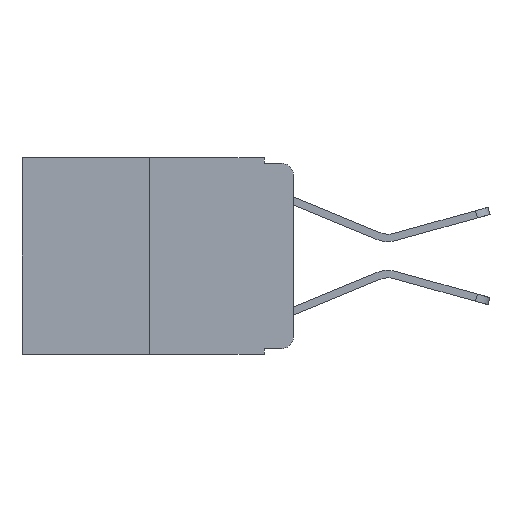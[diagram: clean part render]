
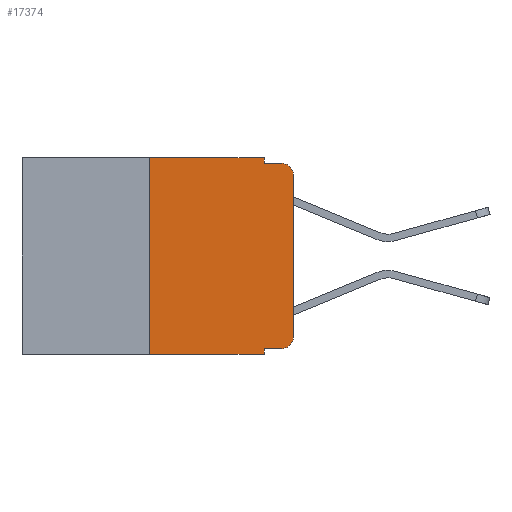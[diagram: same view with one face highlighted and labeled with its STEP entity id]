
A CAD part, left-side view. The second image highlights one B-rep face of the part: STEP entity #17374.
In plain terms, the highlighted planar face has unit normal (-1, 0, 0).
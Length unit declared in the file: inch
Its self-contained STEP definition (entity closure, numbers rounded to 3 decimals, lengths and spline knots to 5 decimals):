
#26 = VECTOR ( 'NONE', #16682, 39.37008 ) ;
#114 = ORIENTED_EDGE ( 'NONE', *, *, #17604, .T. ) ;
#159 = CARTESIAN_POINT ( 'NONE',  ( 0., 0., -0.313 ) ) ;
#179 = ORIENTED_EDGE ( 'NONE', *, *, #16537, .F. ) ;
#199 = ORIENTED_EDGE ( 'NONE', *, *, #10987, .F. ) ;
#278 = ORIENTED_EDGE ( 'NONE', *, *, #18853, .F. ) ;
#306 = ORIENTED_EDGE ( 'NONE', *, *, #9912, .F. ) ;
#359 = ORIENTED_EDGE ( 'NONE', *, *, #1829, .T. ) ;
#443 = ORIENTED_EDGE ( 'NONE', *, *, #5416, .F. ) ;
#446 = ORIENTED_EDGE ( 'NONE', *, *, #4270, .T. ) ;
#464 = ORIENTED_EDGE ( 'NONE', *, *, #3202, .T. ) ;
#810 = ORIENTED_EDGE ( 'NONE', *, *, #19735, .T. ) ;
#1622 = VECTOR ( 'NONE', #2450, 39.37008 ) ;
#1743 = EDGE_LOOP ( 'NONE', ( #810, #114, #179, #199, #278, #306, #359, #443, #446, #464 ) ) ;
#1779 = CARTESIAN_POINT ( 'NONE',  ( 0., 0.051, 0. ) ) ;
#1829 = EDGE_CURVE ( 'NONE', #2483, #19788, #2662, .T. ) ;
#2140 = VECTOR ( 'NONE', #10029, 39.37008 ) ;
#2376 = VERTEX_POINT ( 'NONE', #14789 ) ;
#2450 = DIRECTION ( 'NONE',  ( 0., 0., -1. ) ) ;
#2455 = VECTOR ( 'NONE', #16071, 39.37008 ) ;
#2483 = VERTEX_POINT ( 'NONE', #8677 ) ;
#2662 = LINE ( 'NONE', #11965, #2140 ) ;
#2798 = CARTESIAN_POINT ( 'NONE',  ( 0., 0.051, -0.343 ) ) ;
#2888 = VECTOR ( 'NONE', #16317, 39.37008 ) ;
#2949 = VECTOR ( 'NONE', #7660, 39.37008 ) ;
#3091 = VECTOR ( 'NONE', #15875, 39.37008 ) ;
#3202 = EDGE_CURVE ( 'NONE', #2376, #14727, #15527, .T. ) ;
#3208 = LINE ( 'NONE', #10750, #1622 ) ;
#3642 = CARTESIAN_POINT ( 'NONE',  ( 0., 0., -0.03 ) ) ;
#4011 = LINE ( 'NONE', #11694, #26 ) ;
#4270 = EDGE_CURVE ( 'NONE', #6113, #2376, #15708, .T. ) ;
#4617 = CARTESIAN_POINT ( 'NONE',  ( 0., 0.051, -0.333 ) ) ;
#4711 = DIRECTION ( 'NONE',  ( -1., 0., 0. ) ) ;
#5019 = CARTESIAN_POINT ( 'NONE',  ( 0., 0.473, 0. ) ) ;
#5416 = EDGE_CURVE ( 'NONE', #6113, #19788, #3208, .T. ) ;
#5588 = DIRECTION ( 'NONE',  ( -1., 0., 0. ) ) ;
#5837 = DIRECTION ( 'NONE',  ( 0., -1., 0. ) ) ;
#5843 = CARTESIAN_POINT ( 'NONE',  ( 0., 0.051, 0. ) ) ;
#6113 = VERTEX_POINT ( 'NONE', #4617 ) ;
#6735 = DIRECTION ( 'NONE',  ( 0., 0., -1. ) ) ;
#7368 = LINE ( 'NONE', #14001, #2949 ) ;
#7494 = VERTEX_POINT ( 'NONE', #15639 ) ;
#7660 = DIRECTION ( 'NONE',  ( 0., 0., 1. ) ) ;
#7739 = VERTEX_POINT ( 'NONE', #21065 ) ;
#7992 = CIRCLE ( 'NONE', #11312, 0.02 ) ;
#8677 = CARTESIAN_POINT ( 'NONE',  ( 0., 0.25, -0.343 ) ) ;
#9912 = EDGE_CURVE ( 'NONE', #2483, #7739, #12234, .T. ) ;
#10029 = DIRECTION ( 'NONE',  ( 0., -1., 0. ) ) ;
#10170 = VERTEX_POINT ( 'NONE', #15431 ) ;
#10750 = CARTESIAN_POINT ( 'NONE',  ( 0., 0.051, 0. ) ) ;
#10853 = AXIS2_PLACEMENT_3D ( 'NONE', #14683, #4711, #16334 ) ;
#10987 = EDGE_CURVE ( 'NONE', #16914, #10170, #16843, .T. ) ;
#11312 = AXIS2_PLACEMENT_3D ( 'NONE', #15571, #5588, #17185 ) ;
#11694 = CARTESIAN_POINT ( 'NONE',  ( 0., 0.473, 0. ) ) ;
#11965 = CARTESIAN_POINT ( 'NONE',  ( 0., 0.473, -0.343 ) ) ;
#12234 = LINE ( 'NONE', #17927, #2888 ) ;
#13494 = VERTEX_POINT ( 'NONE', #3642 ) ;
#14001 = CARTESIAN_POINT ( 'NONE',  ( 0., 0., 0. ) ) ;
#14683 = CARTESIAN_POINT ( 'NONE',  ( 0., 0.02, -0.313 ) ) ;
#14727 = VERTEX_POINT ( 'NONE', #159 ) ;
#14789 = CARTESIAN_POINT ( 'NONE',  ( 0., 0.02, -0.333 ) ) ;
#15005 = PLANE ( 'NONE',  #19389 ) ;
#15431 = CARTESIAN_POINT ( 'NONE',  ( 0., 0.051, -0.01 ) ) ;
#15527 = CIRCLE ( 'NONE', #10853, 0.02 ) ;
#15571 = CARTESIAN_POINT ( 'NONE',  ( 0., 0.02, -0.03 ) ) ;
#15639 = CARTESIAN_POINT ( 'NONE',  ( 0., 0.02, -0.01 ) ) ;
#15708 = LINE ( 'NONE', #19296, #2455 ) ;
#15778 = LINE ( 'NONE', #15805, #20045 ) ;
#15805 = CARTESIAN_POINT ( 'NONE',  ( 0., 0.051, -0.01 ) ) ;
#15875 = DIRECTION ( 'NONE',  ( 0., 0., -1. ) ) ;
#16071 = DIRECTION ( 'NONE',  ( 0., -1., 0. ) ) ;
#16317 = DIRECTION ( 'NONE',  ( 0., 0., 1. ) ) ;
#16334 = DIRECTION ( 'NONE',  ( 0., 0., -1. ) ) ;
#16537 = EDGE_CURVE ( 'NONE', #10170, #7494, #15778, .T. ) ;
#16644 = DIRECTION ( 'NONE',  ( 1., 0., 0. ) ) ;
#16682 = DIRECTION ( 'NONE',  ( 0., -1., 0. ) ) ;
#16843 = LINE ( 'NONE', #5843, #3091 ) ;
#16914 = VERTEX_POINT ( 'NONE', #1779 ) ;
#17059 = FACE_OUTER_BOUND ( 'NONE', #1743, .T. ) ;
#17185 = DIRECTION ( 'NONE',  ( 0., 0., -1. ) ) ;
#17374 = ADVANCED_FACE ( 'NONE', ( #17059 ), #15005, .F. ) ;
#17604 = EDGE_CURVE ( 'NONE', #13494, #7494, #7992, .T. ) ;
#17927 = CARTESIAN_POINT ( 'NONE',  ( 0., 0.25, 0. ) ) ;
#18853 = EDGE_CURVE ( 'NONE', #7739, #16914, #4011, .T. ) ;
#19296 = CARTESIAN_POINT ( 'NONE',  ( 0., 0.051, -0.333 ) ) ;
#19389 = AXIS2_PLACEMENT_3D ( 'NONE', #5019, #16644, #6735 ) ;
#19735 = EDGE_CURVE ( 'NONE', #14727, #13494, #7368, .T. ) ;
#19788 = VERTEX_POINT ( 'NONE', #2798 ) ;
#20045 = VECTOR ( 'NONE', #5837, 39.37008 ) ;
#21065 = CARTESIAN_POINT ( 'NONE',  ( 0., 0.25, 0. ) ) ;
